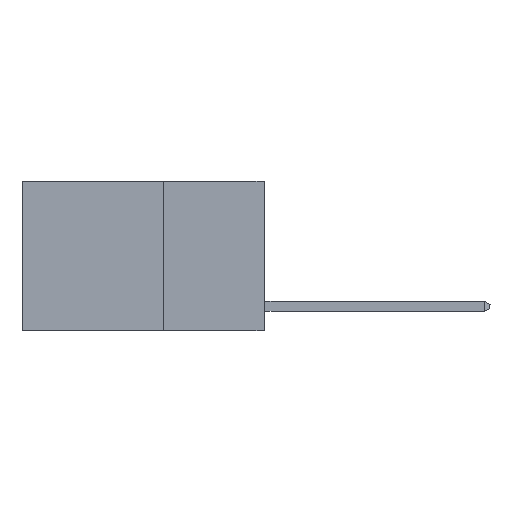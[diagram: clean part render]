
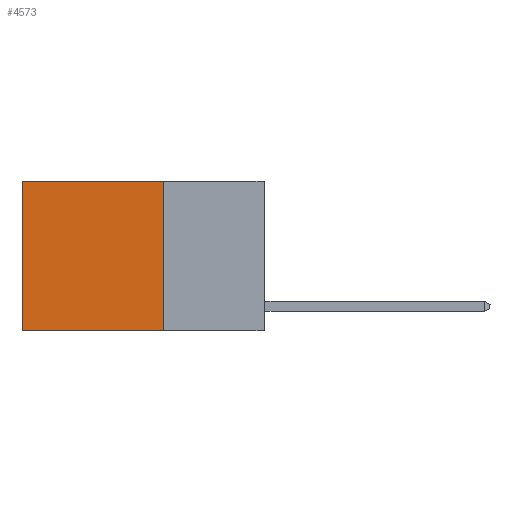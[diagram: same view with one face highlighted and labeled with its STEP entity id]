
A CAD part, left-side view. The second image highlights one B-rep face of the part: STEP entity #4573.
In plain terms, the highlighted planar face has unit normal (-1, 0, 0).
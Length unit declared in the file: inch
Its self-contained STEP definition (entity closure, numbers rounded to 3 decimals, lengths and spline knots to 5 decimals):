
#860 = VECTOR ( 'NONE', #4504, 39.37008 ) ;
#888 = CARTESIAN_POINT ( 'NONE',  ( 0.2625, 0.25, -0.37 ) ) ;
#917 = DIRECTION ( 'NONE',  ( 0., 0., -1. ) ) ;
#1527 = CARTESIAN_POINT ( 'NONE',  ( 0.2625, 0.6, 0. ) ) ;
#1764 = LINE ( 'NONE', #8949, #860 ) ;
#2427 = CARTESIAN_POINT ( 'NONE',  ( 0.2625, 0.25, 0. ) ) ;
#2737 = ORIENTED_EDGE ( 'NONE', *, *, #11333, .F. ) ;
#2741 = DIRECTION ( 'NONE',  ( 0., 0., -1. ) ) ;
#2768 = FACE_OUTER_BOUND ( 'NONE', #6699, .T. ) ;
#2951 = EDGE_CURVE ( 'NONE', #5606, #5875, #14168, .T. ) ;
#3780 = DIRECTION ( 'NONE',  ( 1., 0., 0. ) ) ;
#3785 = LINE ( 'NONE', #7091, #13998 ) ;
#4504 = DIRECTION ( 'NONE',  ( 0., 0., -1. ) ) ;
#4537 = ORIENTED_EDGE ( 'NONE', *, *, #11137, .T. ) ;
#4573 = ADVANCED_FACE ( 'NONE', ( #2768 ), #8486, .F. ) ;
#4583 = ORIENTED_EDGE ( 'NONE', *, *, #2951, .T. ) ;
#5606 = VERTEX_POINT ( 'NONE', #1527 ) ;
#5875 = VERTEX_POINT ( 'NONE', #11563 ) ;
#6376 = CARTESIAN_POINT ( 'NONE',  ( 0.2625, 0.6, 0. ) ) ;
#6699 = EDGE_LOOP ( 'NONE', ( #4583, #11790, #2737, #4537 ) ) ;
#7074 = VECTOR ( 'NONE', #10466, 39.37008 ) ;
#7091 = CARTESIAN_POINT ( 'NONE',  ( 0.2625, 0.25, 0. ) ) ;
#7397 = CARTESIAN_POINT ( 'NONE',  ( 0.2625, 0.25, 0. ) ) ;
#8311 = DIRECTION ( 'NONE',  ( 0., 1., 0. ) ) ;
#8334 = AXIS2_PLACEMENT_3D ( 'NONE', #7397, #3780, #2741 ) ;
#8486 = PLANE ( 'NONE',  #8334 ) ;
#8949 = CARTESIAN_POINT ( 'NONE',  ( 0.2625, 0.25, 0. ) ) ;
#9292 = CARTESIAN_POINT ( 'NONE',  ( 0.2625, 0.25, -0.37 ) ) ;
#9830 = EDGE_CURVE ( 'NONE', #13835, #5875, #13537, .T. ) ;
#10466 = DIRECTION ( 'NONE',  ( 0., 1., 0. ) ) ;
#11137 = EDGE_CURVE ( 'NONE', #11173, #5606, #3785, .T. ) ;
#11173 = VERTEX_POINT ( 'NONE', #2427 ) ;
#11333 = EDGE_CURVE ( 'NONE', #11173, #13835, #1764, .T. ) ;
#11563 = CARTESIAN_POINT ( 'NONE',  ( 0.2625, 0.6, -0.37 ) ) ;
#11774 = VECTOR ( 'NONE', #917, 39.37008 ) ;
#11790 = ORIENTED_EDGE ( 'NONE', *, *, #9830, .F. ) ;
#13537 = LINE ( 'NONE', #9292, #7074 ) ;
#13835 = VERTEX_POINT ( 'NONE', #888 ) ;
#13998 = VECTOR ( 'NONE', #8311, 39.37008 ) ;
#14168 = LINE ( 'NONE', #6376, #11774 ) ;
